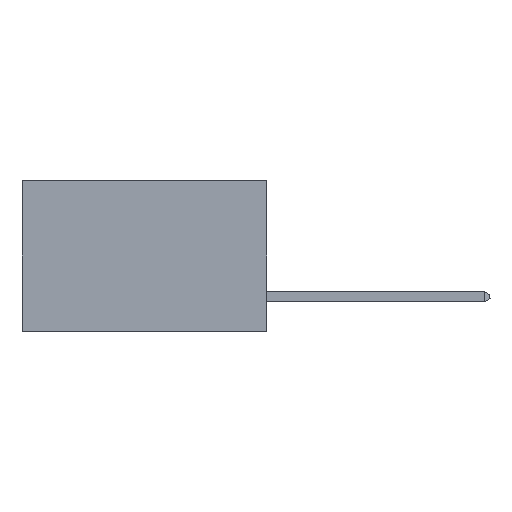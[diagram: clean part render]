
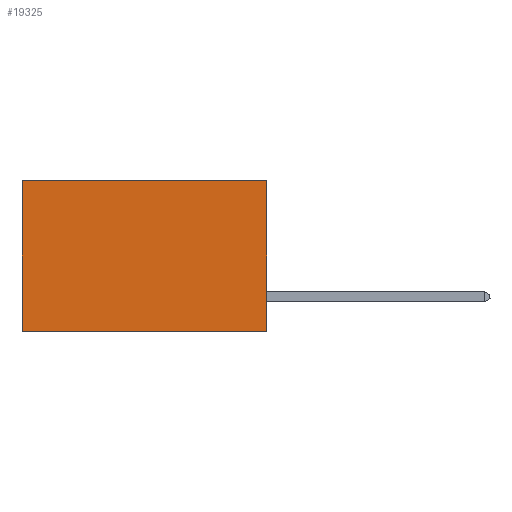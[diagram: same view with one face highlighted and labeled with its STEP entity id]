
A CAD part, left-side view. The second image highlights one B-rep face of the part: STEP entity #19325.
In plain terms, the highlighted planar face has unit normal (-1, 0, 0).
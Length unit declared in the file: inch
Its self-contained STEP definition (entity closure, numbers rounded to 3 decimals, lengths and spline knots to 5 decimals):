
#1924 = ORIENTED_EDGE ( 'NONE', *, *, #14746, .T. ) ;
#3302 = CARTESIAN_POINT ( 'NONE',  ( 0.2875, 0., 0. ) ) ;
#3849 = CARTESIAN_POINT ( 'NONE',  ( 0.2875, 0.6, 0. ) ) ;
#9122 = CARTESIAN_POINT ( 'NONE',  ( 0.2875, 0., 0. ) ) ;
#9192 = ORIENTED_EDGE ( 'NONE', *, *, #14445, .F. ) ;
#9764 = VERTEX_POINT ( 'NONE', #30904 ) ;
#10598 = VECTOR ( 'NONE', #15454, 39.37008 ) ;
#11090 = AXIS2_PLACEMENT_3D ( 'NONE', #29097, #22027, #36625 ) ;
#12068 = CARTESIAN_POINT ( 'NONE',  ( 0.2875, 0., -0.37 ) ) ;
#14011 = DIRECTION ( 'NONE',  ( 0., 1., 0. ) ) ;
#14445 = EDGE_CURVE ( 'NONE', #43767, #38186, #19923, .T. ) ;
#14746 = EDGE_CURVE ( 'NONE', #34962, #9764, #24856, .T. ) ;
#15421 = LINE ( 'NONE', #9122, #32981 ) ;
#15454 = DIRECTION ( 'NONE',  ( 0., 1., 0. ) ) ;
#16770 = ORIENTED_EDGE ( 'NONE', *, *, #43766, .F. ) ;
#18401 = CARTESIAN_POINT ( 'NONE',  ( 0.2875, 0.6, -0.37 ) ) ;
#18497 = PLANE ( 'NONE',  #11090 ) ;
#18827 = CARTESIAN_POINT ( 'NONE',  ( 0.2875, 0., -0.37 ) ) ;
#19325 = ADVANCED_FACE ( 'NONE', ( #42353 ), #18497, .F. ) ;
#19923 = LINE ( 'NONE', #18827, #10598 ) ;
#21365 = VECTOR ( 'NONE', #28426, 39.37008 ) ;
#22027 = DIRECTION ( 'NONE',  ( 1., 0., 0. ) ) ;
#24445 = CARTESIAN_POINT ( 'NONE',  ( 0.2875, 0., 0. ) ) ;
#24856 = LINE ( 'NONE', #24445, #41369 ) ;
#26732 = EDGE_CURVE ( 'NONE', #9764, #38186, #28518, .T. ) ;
#28426 = DIRECTION ( 'NONE',  ( 0., 0., -1. ) ) ;
#28518 = LINE ( 'NONE', #3849, #21365 ) ;
#28734 = EDGE_LOOP ( 'NONE', ( #41239, #9192, #16770, #1924 ) ) ;
#29097 = CARTESIAN_POINT ( 'NONE',  ( 0.2875, 0., 0. ) ) ;
#30904 = CARTESIAN_POINT ( 'NONE',  ( 0.2875, 0.6, 0. ) ) ;
#32981 = VECTOR ( 'NONE', #43702, 39.37008 ) ;
#34962 = VERTEX_POINT ( 'NONE', #3302 ) ;
#36625 = DIRECTION ( 'NONE',  ( 0., 0., -1. ) ) ;
#38186 = VERTEX_POINT ( 'NONE', #18401 ) ;
#41239 = ORIENTED_EDGE ( 'NONE', *, *, #26732, .T. ) ;
#41369 = VECTOR ( 'NONE', #14011, 39.37008 ) ;
#42353 = FACE_OUTER_BOUND ( 'NONE', #28734, .T. ) ;
#43702 = DIRECTION ( 'NONE',  ( 0., 0., -1. ) ) ;
#43766 = EDGE_CURVE ( 'NONE', #34962, #43767, #15421, .T. ) ;
#43767 = VERTEX_POINT ( 'NONE', #12068 ) ;
